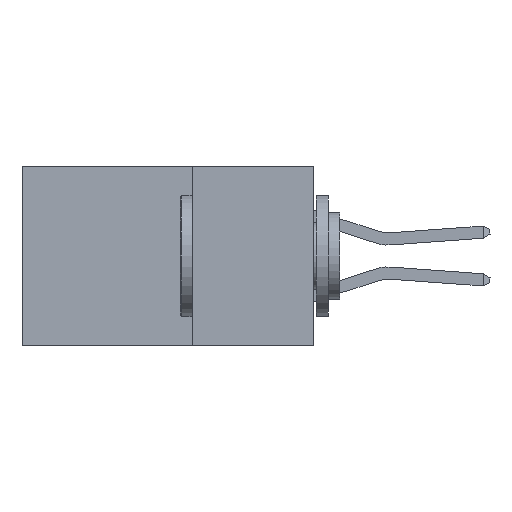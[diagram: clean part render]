
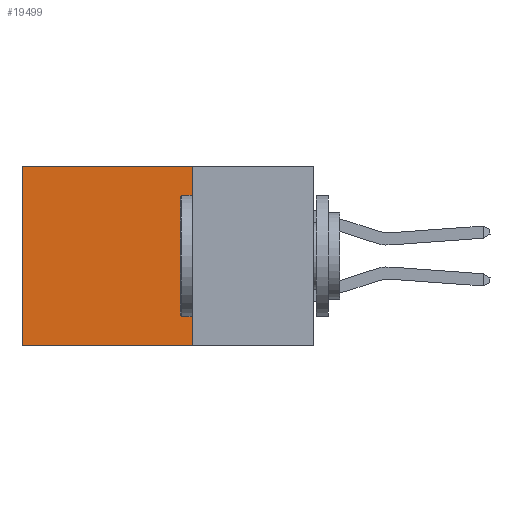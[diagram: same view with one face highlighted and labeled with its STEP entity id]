
A CAD part, left-side view. The second image highlights one B-rep face of the part: STEP entity #19499.
In plain terms, the highlighted planar face has unit normal (-1, 0, 0).
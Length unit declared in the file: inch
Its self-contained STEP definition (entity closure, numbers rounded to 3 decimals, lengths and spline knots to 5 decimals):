
#259 = ORIENTED_EDGE ( 'NONE', *, *, #832, .F. ) ;
#717 = PLANE ( 'NONE',  #16697 ) ;
#832 = EDGE_CURVE ( 'NONE', #2551, #1412, #20222, .T. ) ;
#1412 = VERTEX_POINT ( 'NONE', #16257 ) ;
#2098 = VECTOR ( 'NONE', #13230, 39.37008 ) ;
#2551 = VERTEX_POINT ( 'NONE', #18724 ) ;
#2714 = LINE ( 'NONE', #16851, #2098 ) ;
#3964 = VECTOR ( 'NONE', #14542, 39.37008 ) ;
#5207 = VERTEX_POINT ( 'NONE', #7750 ) ;
#5416 = CARTESIAN_POINT ( 'NONE',  ( 0.2875, 0.6, 0. ) ) ;
#5502 = VECTOR ( 'NONE', #7380, 39.37008 ) ;
#5705 = DIRECTION ( 'NONE',  ( 0., 0., -1. ) ) ;
#6436 = EDGE_CURVE ( 'NONE', #5207, #13276, #20230, .T. ) ;
#7045 = ORIENTED_EDGE ( 'NONE', *, *, #18416, .T. ) ;
#7281 = CARTESIAN_POINT ( 'NONE',  ( 0.2875, 0.25, 0. ) ) ;
#7380 = DIRECTION ( 'NONE',  ( 0., 0., -1. ) ) ;
#7750 = CARTESIAN_POINT ( 'NONE',  ( 0.2875, 0.6, 0. ) ) ;
#8460 = CARTESIAN_POINT ( 'NONE',  ( 0.2875, 0.25, 0. ) ) ;
#10334 = DIRECTION ( 'NONE',  ( 0., 0., -1. ) ) ;
#12730 = CARTESIAN_POINT ( 'NONE',  ( 0.2875, 0.25, 0. ) ) ;
#13230 = DIRECTION ( 'NONE',  ( 0., 1., 0. ) ) ;
#13276 = VERTEX_POINT ( 'NONE', #22834 ) ;
#14281 = EDGE_LOOP ( 'NONE', ( #15727, #17498, #259, #7045 ) ) ;
#14542 = DIRECTION ( 'NONE',  ( 0., 1., 0. ) ) ;
#15386 = EDGE_CURVE ( 'NONE', #1412, #13276, #2714, .T. ) ;
#15727 = ORIENTED_EDGE ( 'NONE', *, *, #6436, .T. ) ;
#16257 = CARTESIAN_POINT ( 'NONE',  ( 0.2875, 0.25, -0.37 ) ) ;
#16697 = AXIS2_PLACEMENT_3D ( 'NONE', #8460, #21203, #10334 ) ;
#16851 = CARTESIAN_POINT ( 'NONE',  ( 0.2875, 0.25, -0.37 ) ) ;
#17498 = ORIENTED_EDGE ( 'NONE', *, *, #15386, .F. ) ;
#18416 = EDGE_CURVE ( 'NONE', #2551, #5207, #18791, .T. ) ;
#18460 = FACE_OUTER_BOUND ( 'NONE', #14281, .T. ) ;
#18724 = CARTESIAN_POINT ( 'NONE',  ( 0.2875, 0.25, 0. ) ) ;
#18791 = LINE ( 'NONE', #12730, #3964 ) ;
#19499 = ADVANCED_FACE ( 'NONE', ( #18460 ), #717, .F. ) ;
#19662 = VECTOR ( 'NONE', #5705, 39.37008 ) ;
#20222 = LINE ( 'NONE', #7281, #19662 ) ;
#20230 = LINE ( 'NONE', #5416, #5502 ) ;
#21203 = DIRECTION ( 'NONE',  ( 1., 0., 0. ) ) ;
#22834 = CARTESIAN_POINT ( 'NONE',  ( 0.2875, 0.6, -0.37 ) ) ;
